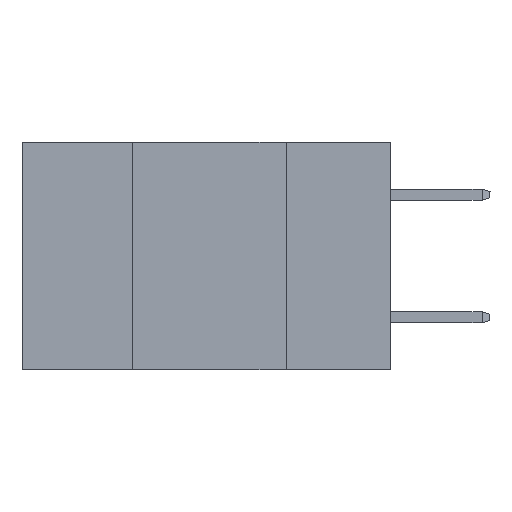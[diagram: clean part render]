
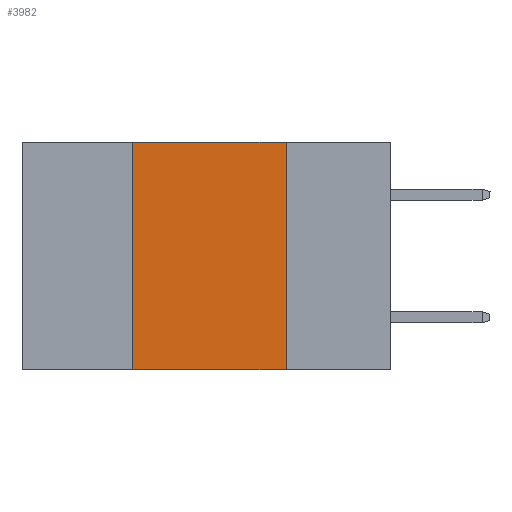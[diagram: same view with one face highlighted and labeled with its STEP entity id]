
A CAD part, left-side view. The second image highlights one B-rep face of the part: STEP entity #3982.
In plain terms, the highlighted planar face has unit normal (-1, 0, 0).
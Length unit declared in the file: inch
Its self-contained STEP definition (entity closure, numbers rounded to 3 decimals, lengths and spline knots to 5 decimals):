
#581 = LINE ( 'NONE', #7568, #23914 ) ;
#1036 = VERTEX_POINT ( 'NONE', #12557 ) ;
#1387 = LINE ( 'NONE', #25145, #16101 ) ;
#1766 = EDGE_CURVE ( 'NONE', #15813, #1036, #6119, .T. ) ;
#2280 = PLANE ( 'NONE',  #13780 ) ;
#3061 = VERTEX_POINT ( 'NONE', #7327 ) ;
#3982 = ADVANCED_FACE ( 'NONE', ( #24686 ), #2280, .F. ) ;
#4377 = CARTESIAN_POINT ( 'NONE',  ( 0., 0.42, 0. ) ) ;
#5558 = ORIENTED_EDGE ( 'NONE', *, *, #6679, .F. ) ;
#6119 = LINE ( 'NONE', #7950, #15891 ) ;
#6172 = DIRECTION ( 'NONE',  ( 0., -1., 0. ) ) ;
#6237 = CARTESIAN_POINT ( 'NONE',  ( 0., 0.6, 0. ) ) ;
#6449 = VECTOR ( 'NONE', #20330, 39.37008 ) ;
#6679 = EDGE_CURVE ( 'NONE', #1036, #3061, #11639, .T. ) ;
#7327 = CARTESIAN_POINT ( 'NONE',  ( 0., 0.17, -0.37 ) ) ;
#7568 = CARTESIAN_POINT ( 'NONE',  ( 0., 0.6, -0.37 ) ) ;
#7908 = EDGE_LOOP ( 'NONE', ( #5558, #22184, #14445, #19423 ) ) ;
#7950 = CARTESIAN_POINT ( 'NONE',  ( 0., 0.6, 0. ) ) ;
#8188 = DIRECTION ( 'NONE',  ( 1., 0., 0. ) ) ;
#10147 = DIRECTION ( 'NONE',  ( 0., 0., -1. ) ) ;
#10561 = EDGE_CURVE ( 'NONE', #17642, #15813, #1387, .T. ) ;
#11485 = DIRECTION ( 'NONE',  ( 0., 0., 1. ) ) ;
#11639 = LINE ( 'NONE', #19750, #6449 ) ;
#12557 = CARTESIAN_POINT ( 'NONE',  ( 0., 0.17, 0. ) ) ;
#13780 = AXIS2_PLACEMENT_3D ( 'NONE', #6237, #8188, #10147 ) ;
#14445 = ORIENTED_EDGE ( 'NONE', *, *, #10561, .F. ) ;
#15413 = CARTESIAN_POINT ( 'NONE',  ( 0., 0.42, -0.37 ) ) ;
#15813 = VERTEX_POINT ( 'NONE', #4377 ) ;
#15891 = VECTOR ( 'NONE', #6172, 39.37008 ) ;
#16101 = VECTOR ( 'NONE', #11485, 39.37008 ) ;
#17420 = DIRECTION ( 'NONE',  ( 0., -1., 0. ) ) ;
#17642 = VERTEX_POINT ( 'NONE', #15413 ) ;
#19423 = ORIENTED_EDGE ( 'NONE', *, *, #22089, .T. ) ;
#19750 = CARTESIAN_POINT ( 'NONE',  ( 0., 0.17, 0. ) ) ;
#20330 = DIRECTION ( 'NONE',  ( 0., 0., -1. ) ) ;
#22089 = EDGE_CURVE ( 'NONE', #17642, #3061, #581, .T. ) ;
#22184 = ORIENTED_EDGE ( 'NONE', *, *, #1766, .F. ) ;
#23914 = VECTOR ( 'NONE', #17420, 39.37008 ) ;
#24686 = FACE_OUTER_BOUND ( 'NONE', #7908, .T. ) ;
#25145 = CARTESIAN_POINT ( 'NONE',  ( 0., 0.42, 0. ) ) ;
